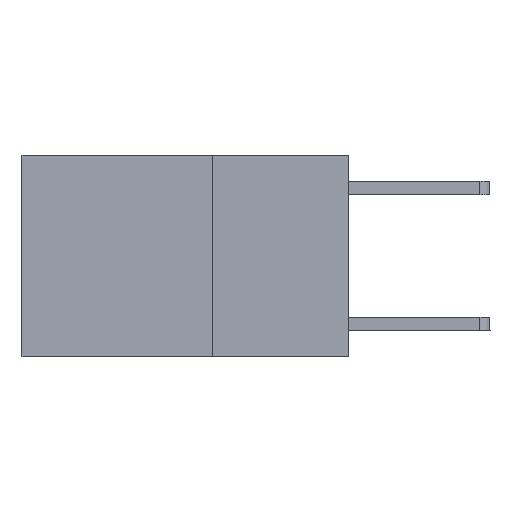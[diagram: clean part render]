
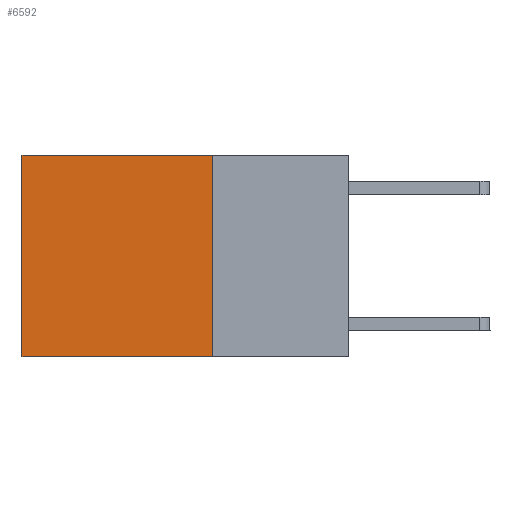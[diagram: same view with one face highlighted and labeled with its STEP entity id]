
A CAD part, left-side view. The second image highlights one B-rep face of the part: STEP entity #6592.
In plain terms, the highlighted planar face has unit normal (-1, 0, 0).
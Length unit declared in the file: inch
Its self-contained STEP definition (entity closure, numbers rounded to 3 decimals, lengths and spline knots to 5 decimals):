
#105 = CARTESIAN_POINT ( 'NONE',  ( 0.2625, 0.25, 0. ) ) ;
#274 = VECTOR ( 'NONE', #10566, 39.37008 ) ;
#364 = VERTEX_POINT ( 'NONE', #3525 ) ;
#696 = VECTOR ( 'NONE', #5919, 39.37008 ) ;
#1470 = EDGE_CURVE ( 'NONE', #9870, #6114, #5353, .T. ) ;
#1504 = AXIS2_PLACEMENT_3D ( 'NONE', #5706, #2993, #9363 ) ;
#2180 = CARTESIAN_POINT ( 'NONE',  ( 0.2625, 0.25, -0.37 ) ) ;
#2418 = CARTESIAN_POINT ( 'NONE',  ( 0.2625, 0.25, 0. ) ) ;
#2932 = VECTOR ( 'NONE', #5076, 39.37008 ) ;
#2993 = DIRECTION ( 'NONE',  ( 1., 0., 0. ) ) ;
#3262 = EDGE_LOOP ( 'NONE', ( #8747, #8835, #8885, #8955 ) ) ;
#3291 = CARTESIAN_POINT ( 'NONE',  ( 0.2625, 0.6, -0.37 ) ) ;
#3391 = LINE ( 'NONE', #105, #3684 ) ;
#3525 = CARTESIAN_POINT ( 'NONE',  ( 0.2625, 0.6, 0. ) ) ;
#3621 = VERTEX_POINT ( 'NONE', #2418 ) ;
#3684 = VECTOR ( 'NONE', #9357, 39.37008 ) ;
#4977 = CARTESIAN_POINT ( 'NONE',  ( 0.2625, 0.6, 0. ) ) ;
#5076 = DIRECTION ( 'NONE',  ( 0., 1., 0. ) ) ;
#5234 = LINE ( 'NONE', #9635, #274 ) ;
#5353 = LINE ( 'NONE', #6938, #2932 ) ;
#5706 = CARTESIAN_POINT ( 'NONE',  ( 0.2625, 0.25, 0. ) ) ;
#5919 = DIRECTION ( 'NONE',  ( 0., 0., -1. ) ) ;
#6114 = VERTEX_POINT ( 'NONE', #3291 ) ;
#6431 = FACE_OUTER_BOUND ( 'NONE', #3262, .T. ) ;
#6592 = ADVANCED_FACE ( 'NONE', ( #6431 ), #8465, .F. ) ;
#6938 = CARTESIAN_POINT ( 'NONE',  ( 0.2625, 0.25, -0.37 ) ) ;
#8068 = EDGE_CURVE ( 'NONE', #3621, #9870, #5234, .T. ) ;
#8075 = LINE ( 'NONE', #4977, #696 ) ;
#8465 = PLANE ( 'NONE',  #1504 ) ;
#8502 = EDGE_CURVE ( 'NONE', #3621, #364, #3391, .T. ) ;
#8747 = ORIENTED_EDGE ( 'NONE', *, *, #11125, .T. ) ;
#8835 = ORIENTED_EDGE ( 'NONE', *, *, #1470, .F. ) ;
#8885 = ORIENTED_EDGE ( 'NONE', *, *, #8068, .F. ) ;
#8955 = ORIENTED_EDGE ( 'NONE', *, *, #8502, .T. ) ;
#9357 = DIRECTION ( 'NONE',  ( 0., 1., 0. ) ) ;
#9363 = DIRECTION ( 'NONE',  ( 0., 0., -1. ) ) ;
#9635 = CARTESIAN_POINT ( 'NONE',  ( 0.2625, 0.25, 0. ) ) ;
#9870 = VERTEX_POINT ( 'NONE', #2180 ) ;
#10566 = DIRECTION ( 'NONE',  ( 0., 0., -1. ) ) ;
#11125 = EDGE_CURVE ( 'NONE', #364, #6114, #8075, .T. ) ;
